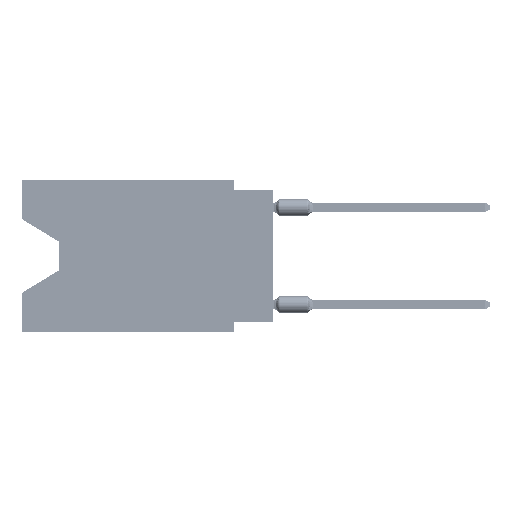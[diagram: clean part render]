
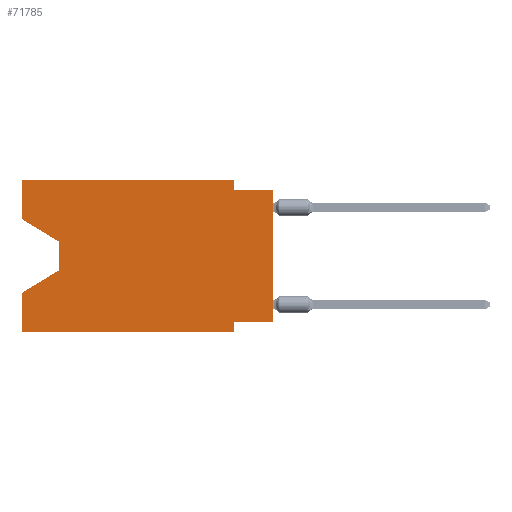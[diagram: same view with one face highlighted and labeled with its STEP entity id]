
A CAD part, left-side view. The second image highlights one B-rep face of the part: STEP entity #71785.
In plain terms, the highlighted planar face has unit normal (-1, 0, 0).
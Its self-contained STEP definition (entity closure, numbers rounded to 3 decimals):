
#2779 = VERTEX_POINT ( 'NONE', #11308 ) ;
#4232 = DIRECTION ( 'NONE',  ( 0., -1., 0. ) ) ;
#4533 = ORIENTED_EDGE ( 'NONE', *, *, #8541, .F. ) ;
#4736 = CARTESIAN_POINT ( 'NONE',  ( 0., 16.383, 0. ) ) ;
#4921 = VECTOR ( 'NONE', #19791, 1000. ) ;
#5700 = LINE ( 'NONE', #28735, #28820 ) ;
#5800 = VERTEX_POINT ( 'NONE', #12480 ) ;
#6807 = EDGE_CURVE ( 'NONE', #60641, #51072, #21240, .T. ) ;
#7354 = LINE ( 'NONE', #54548, #34077 ) ;
#8541 = EDGE_CURVE ( 'NONE', #66427, #37885, #17349, .T. ) ;
#8842 = DIRECTION ( 'NONE',  ( 0., -0.855, -0.519 ) ) ;
#10584 = DIRECTION ( 'NONE',  ( 0., 0.855, -0.519 ) ) ;
#10868 = ORIENTED_EDGE ( 'NONE', *, *, #43114, .T. ) ;
#11036 = VERTEX_POINT ( 'NONE', #61746 ) ;
#11308 = CARTESIAN_POINT ( 'NONE',  ( 0., 13.97, -4.013 ) ) ;
#11746 = DIRECTION ( 'NONE',  ( 0., 0., -1. ) ) ;
#12480 = CARTESIAN_POINT ( 'NONE',  ( 0., 13.97, -5.893 ) ) ;
#12528 = ORIENTED_EDGE ( 'NONE', *, *, #51895, .F. ) ;
#14223 = CARTESIAN_POINT ( 'NONE',  ( 0., 16.383, -7.36 ) ) ;
#15057 = ORIENTED_EDGE ( 'NONE', *, *, #37632, .F. ) ;
#15229 = ORIENTED_EDGE ( 'NONE', *, *, #43315, .F. ) ;
#15266 = LINE ( 'NONE', #67379, #27633 ) ;
#17349 = LINE ( 'NONE', #45292, #27519 ) ;
#17696 = ORIENTED_EDGE ( 'NONE', *, *, #74041, .F. ) ;
#18219 = CARTESIAN_POINT ( 'NONE',  ( 0., 16.383, -9.906 ) ) ;
#18314 = ORIENTED_EDGE ( 'NONE', *, *, #51468, .F. ) ;
#18393 = VECTOR ( 'NONE', #27570, 1000. ) ;
#19791 = DIRECTION ( 'NONE',  ( 0., 0., -1. ) ) ;
#19995 = CARTESIAN_POINT ( 'NONE',  ( 0., 16.383, 0. ) ) ;
#20243 = EDGE_LOOP ( 'NONE', ( #10868, #23842, #66390, #18314, #68812, #17696, #15229, #64476, #74307, #12528, #15057, #4533 ) ) ;
#20251 = VERTEX_POINT ( 'NONE', #21452 ) ;
#20550 = DIRECTION ( 'NONE',  ( 0., 0., -1. ) ) ;
#21240 = LINE ( 'NONE', #55979, #71830 ) ;
#21452 = CARTESIAN_POINT ( 'NONE',  ( 0., 2.54, 0. ) ) ;
#21912 = CARTESIAN_POINT ( 'NONE',  ( 0., 16.383, 0. ) ) ;
#23842 = ORIENTED_EDGE ( 'NONE', *, *, #55609, .T. ) ;
#24732 = LINE ( 'NONE', #25471, #70271 ) ;
#25471 = CARTESIAN_POINT ( 'NONE',  ( 0., 0., -0.635 ) ) ;
#26769 = FACE_OUTER_BOUND ( 'NONE', #20243, .T. ) ;
#27519 = VECTOR ( 'NONE', #44921, 1000. ) ;
#27570 = DIRECTION ( 'NONE',  ( 0., -1., 0. ) ) ;
#27633 = VECTOR ( 'NONE', #20550, 1000. ) ;
#28735 = CARTESIAN_POINT ( 'NONE',  ( 0., 2.54, -9.906 ) ) ;
#28820 = VECTOR ( 'NONE', #11746, 1000. ) ;
#30372 = CARTESIAN_POINT ( 'NONE',  ( 0., 2.54, -0.635 ) ) ;
#30769 = DIRECTION ( 'NONE',  ( 0., -1., 0. ) ) ;
#32068 = DIRECTION ( 'NONE',  ( 1., 0., 0. ) ) ;
#33619 = VECTOR ( 'NONE', #72382, 1000. ) ;
#34077 = VECTOR ( 'NONE', #47373, 1000. ) ;
#34365 = CARTESIAN_POINT ( 'NONE',  ( 0., 16.383, 0. ) ) ;
#36532 = CARTESIAN_POINT ( 'NONE',  ( 0., 0., -0.635 ) ) ;
#37233 = VECTOR ( 'NONE', #8842, 1000. ) ;
#37534 = CARTESIAN_POINT ( 'NONE',  ( 0., 16.383, -2.546 ) ) ;
#37632 = EDGE_CURVE ( 'NONE', #37885, #20251, #44938, .T. ) ;
#37885 = VERTEX_POINT ( 'NONE', #34365 ) ;
#38279 = LINE ( 'NONE', #72281, #4921 ) ;
#39431 = VERTEX_POINT ( 'NONE', #62659 ) ;
#42977 = VERTEX_POINT ( 'NONE', #30372 ) ;
#43023 = DIRECTION ( 'NONE',  ( 0., 0., -1. ) ) ;
#43114 = EDGE_CURVE ( 'NONE', #66427, #2779, #49601, .T. ) ;
#43315 = EDGE_CURVE ( 'NONE', #11036, #39431, #51826, .T. ) ;
#43961 = VERTEX_POINT ( 'NONE', #14223 ) ;
#44921 = DIRECTION ( 'NONE',  ( 0., 0., 1. ) ) ;
#44938 = LINE ( 'NONE', #21912, #18393 ) ;
#44945 = CARTESIAN_POINT ( 'NONE',  ( 0., 13.97, -5.893 ) ) ;
#45292 = CARTESIAN_POINT ( 'NONE',  ( 0., 16.383, 0. ) ) ;
#47364 = VECTOR ( 'NONE', #10584, 1000. ) ;
#47373 = DIRECTION ( 'NONE',  ( 0., 0., 1. ) ) ;
#48681 = PLANE ( 'NONE',  #51512 ) ;
#49601 = LINE ( 'NONE', #37534, #37233 ) ;
#49877 = LINE ( 'NONE', #44945, #47364 ) ;
#50999 = CARTESIAN_POINT ( 'NONE',  ( 0., 16.383, -2.546 ) ) ;
#51072 = VERTEX_POINT ( 'NONE', #65795 ) ;
#51468 = EDGE_CURVE ( 'NONE', #60641, #43961, #67468, .T. ) ;
#51512 = AXIS2_PLACEMENT_3D ( 'NONE', #19995, #32068, #43023 ) ;
#51826 = LINE ( 'NONE', #52932, #52945 ) ;
#51895 = EDGE_CURVE ( 'NONE', #20251, #42977, #15266, .T. ) ;
#52932 = CARTESIAN_POINT ( 'NONE',  ( 0., 0., -9.271 ) ) ;
#52945 = VECTOR ( 'NONE', #70326, 1000. ) ;
#54548 = CARTESIAN_POINT ( 'NONE',  ( 0., 0., 0. ) ) ;
#55609 = EDGE_CURVE ( 'NONE', #2779, #5800, #38279, .T. ) ;
#55979 = CARTESIAN_POINT ( 'NONE',  ( 0., 16.383, -9.906 ) ) ;
#57896 = EDGE_CURVE ( 'NONE', #42977, #66982, #24732, .T. ) ;
#60363 = EDGE_CURVE ( 'NONE', #11036, #66982, #7354, .T. ) ;
#60641 = VERTEX_POINT ( 'NONE', #18219 ) ;
#61746 = CARTESIAN_POINT ( 'NONE',  ( 0., 0., -9.271 ) ) ;
#62659 = CARTESIAN_POINT ( 'NONE',  ( 0., 2.54, -9.271 ) ) ;
#64476 = ORIENTED_EDGE ( 'NONE', *, *, #60363, .T. ) ;
#65337 = EDGE_CURVE ( 'NONE', #5800, #43961, #49877, .T. ) ;
#65795 = CARTESIAN_POINT ( 'NONE',  ( 0., 2.54, -9.906 ) ) ;
#66390 = ORIENTED_EDGE ( 'NONE', *, *, #65337, .T. ) ;
#66427 = VERTEX_POINT ( 'NONE', #50999 ) ;
#66982 = VERTEX_POINT ( 'NONE', #36532 ) ;
#67379 = CARTESIAN_POINT ( 'NONE',  ( 0., 2.54, 0. ) ) ;
#67468 = LINE ( 'NONE', #4736, #33619 ) ;
#68812 = ORIENTED_EDGE ( 'NONE', *, *, #6807, .T. ) ;
#70271 = VECTOR ( 'NONE', #30769, 1000. ) ;
#70326 = DIRECTION ( 'NONE',  ( 0., 1., 0. ) ) ;
#71785 = ADVANCED_FACE ( 'NONE', ( #26769 ), #48681, .F. ) ;
#71830 = VECTOR ( 'NONE', #4232, 1000. ) ;
#72281 = CARTESIAN_POINT ( 'NONE',  ( 0., 13.97, -4.013 ) ) ;
#72382 = DIRECTION ( 'NONE',  ( 0., 0., 1. ) ) ;
#74041 = EDGE_CURVE ( 'NONE', #39431, #51072, #5700, .T. ) ;
#74307 = ORIENTED_EDGE ( 'NONE', *, *, #57896, .F. ) ;
